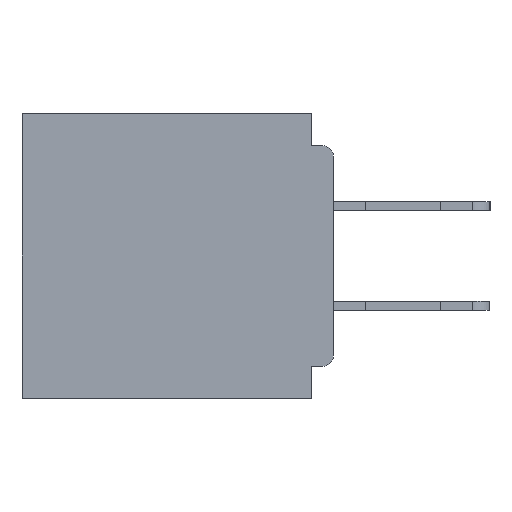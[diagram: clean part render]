
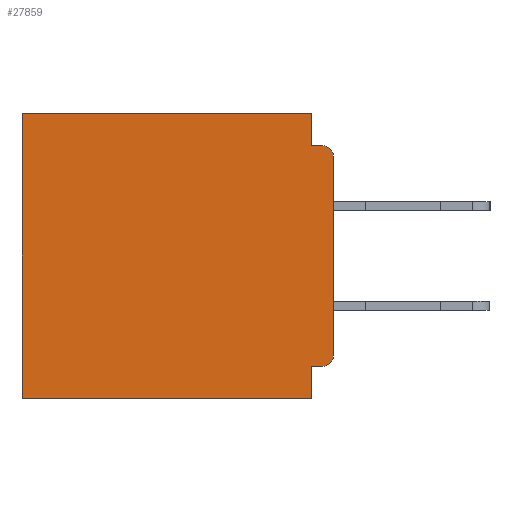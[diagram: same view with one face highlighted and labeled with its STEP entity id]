
A CAD part, left-side view. The second image highlights one B-rep face of the part: STEP entity #27859.
In plain terms, the highlighted planar face has unit normal (-1, 0, 0).
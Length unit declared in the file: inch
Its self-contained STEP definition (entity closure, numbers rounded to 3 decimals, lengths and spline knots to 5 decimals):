
#535 = VECTOR ( 'NONE', #12243, 39.37008 ) ;
#715 = VERTEX_POINT ( 'NONE', #3786 ) ;
#739 = ORIENTED_EDGE ( 'NONE', *, *, #3832, .T. ) ;
#997 = DIRECTION ( 'NONE',  ( 0., 0., -1. ) ) ;
#2430 = ORIENTED_EDGE ( 'NONE', *, *, #18139, .F. ) ;
#3179 = ORIENTED_EDGE ( 'NONE', *, *, #42944, .F. ) ;
#3397 = CARTESIAN_POINT ( 'NONE',  ( 0.3, 0.015, -0.34 ) ) ;
#3786 = CARTESIAN_POINT ( 'NONE',  ( 0.3, 0.031, -0.355 ) ) ;
#3832 = EDGE_CURVE ( 'NONE', #22852, #14120, #15220, .T. ) ;
#4287 = VERTEX_POINT ( 'NONE', #28730 ) ;
#5738 = CARTESIAN_POINT ( 'NONE',  ( 0.3, 0., -0.4 ) ) ;
#5742 = ORIENTED_EDGE ( 'NONE', *, *, #34414, .T. ) ;
#6948 = EDGE_CURVE ( 'NONE', #56632, #6965, #15062, .T. ) ;
#6965 = VERTEX_POINT ( 'NONE', #21066 ) ;
#7620 = LINE ( 'NONE', #5738, #16630 ) ;
#7742 = VECTOR ( 'NONE', #51944, 39.37008 ) ;
#7922 = DIRECTION ( 'NONE',  ( 0., 0., -1. ) ) ;
#9125 = LINE ( 'NONE', #47590, #7742 ) ;
#9281 = FACE_OUTER_BOUND ( 'NONE', #45149, .T. ) ;
#9583 = LINE ( 'NONE', #13804, #41954 ) ;
#9831 = DIRECTION ( 'NONE',  ( 1., 0., 0. ) ) ;
#10188 = DIRECTION ( 'NONE',  ( 0., 0., -1. ) ) ;
#10268 = CARTESIAN_POINT ( 'NONE',  ( 0.3, 0.015, -0.045 ) ) ;
#12243 = DIRECTION ( 'NONE',  ( 0., 0., -1. ) ) ;
#12942 = VERTEX_POINT ( 'NONE', #48364 ) ;
#13123 = AXIS2_PLACEMENT_3D ( 'NONE', #17853, #48549, #22221 ) ;
#13804 = CARTESIAN_POINT ( 'NONE',  ( 0.3, 0., -0.045 ) ) ;
#14120 = VERTEX_POINT ( 'NONE', #25967 ) ;
#15062 = CIRCLE ( 'NONE', #40680, 0.015 ) ;
#15220 = LINE ( 'NONE', #31015, #48896 ) ;
#15748 = ORIENTED_EDGE ( 'NONE', *, *, #42782, .T. ) ;
#16630 = VECTOR ( 'NONE', #10188, 39.37008 ) ;
#17853 = CARTESIAN_POINT ( 'NONE',  ( 0.3, 0.015, -0.06 ) ) ;
#18139 = EDGE_CURVE ( 'NONE', #56632, #715, #43212, .T. ) ;
#18301 = DIRECTION ( 'NONE',  ( 0., -1., 0. ) ) ;
#18500 = CARTESIAN_POINT ( 'NONE',  ( 0.3, 0., -0.355 ) ) ;
#18995 = CARTESIAN_POINT ( 'NONE',  ( 0.3, 0., -0.4 ) ) ;
#20070 = CARTESIAN_POINT ( 'NONE',  ( 0.3, 0.031, 0. ) ) ;
#21066 = CARTESIAN_POINT ( 'NONE',  ( 0.3, 0., -0.34 ) ) ;
#21254 = VERTEX_POINT ( 'NONE', #28806 ) ;
#22221 = DIRECTION ( 'NONE',  ( 0., 0., -1. ) ) ;
#22852 = VERTEX_POINT ( 'NONE', #22892 ) ;
#22892 = CARTESIAN_POINT ( 'NONE',  ( 0.3, 0.437, 0. ) ) ;
#24108 = LINE ( 'NONE', #18995, #44732 ) ;
#25967 = CARTESIAN_POINT ( 'NONE',  ( 0.3, 0.437, -0.4 ) ) ;
#27859 = ADVANCED_FACE ( 'NONE', ( #9281 ), #53790, .F. ) ;
#28730 = CARTESIAN_POINT ( 'NONE',  ( 0.3, 0.031, -0.045 ) ) ;
#28806 = CARTESIAN_POINT ( 'NONE',  ( 0.3, 0.031, -0.4 ) ) ;
#28920 = LINE ( 'NONE', #20070, #39244 ) ;
#31006 = CIRCLE ( 'NONE', #13123, 0.015 ) ;
#31015 = CARTESIAN_POINT ( 'NONE',  ( 0.3, 0.437, -0.4 ) ) ;
#31460 = DIRECTION ( 'NONE',  ( 0., 0., -1. ) ) ;
#31573 = VECTOR ( 'NONE', #40370, 39.37008 ) ;
#33031 = CARTESIAN_POINT ( 'NONE',  ( 0.3, 0.031, 0. ) ) ;
#34342 = DIRECTION ( 'NONE',  ( -1., 0., 0. ) ) ;
#34414 = EDGE_CURVE ( 'NONE', #52807, #22852, #9125, .T. ) ;
#35971 = EDGE_CURVE ( 'NONE', #52807, #4287, #28920, .T. ) ;
#36337 = EDGE_CURVE ( 'NONE', #4287, #50828, #9583, .T. ) ;
#36774 = ORIENTED_EDGE ( 'NONE', *, *, #35971, .F. ) ;
#37721 = DIRECTION ( 'NONE',  ( 0., 0., -1. ) ) ;
#38442 = CARTESIAN_POINT ( 'NONE',  ( 0.3, 0.015, -0.355 ) ) ;
#38523 = ORIENTED_EDGE ( 'NONE', *, *, #36337, .F. ) ;
#39244 = VECTOR ( 'NONE', #37721, 39.37008 ) ;
#40117 = AXIS2_PLACEMENT_3D ( 'NONE', #49453, #9831, #997 ) ;
#40370 = DIRECTION ( 'NONE',  ( 0., 1., 0. ) ) ;
#40680 = AXIS2_PLACEMENT_3D ( 'NONE', #3397, #34342, #7922 ) ;
#41954 = VECTOR ( 'NONE', #18301, 39.37008 ) ;
#42782 = EDGE_CURVE ( 'NONE', #12942, #50828, #31006, .T. ) ;
#42944 = EDGE_CURVE ( 'NONE', #21254, #14120, #24108, .T. ) ;
#43212 = LINE ( 'NONE', #18500, #31573 ) ;
#43599 = EDGE_CURVE ( 'NONE', #12942, #6965, #7620, .T. ) ;
#44732 = VECTOR ( 'NONE', #54015, 39.37008 ) ;
#45149 = EDGE_LOOP ( 'NONE', ( #51095, #15748, #38523, #36774, #5742, #739, #3179, #45948, #2430, #57024 ) ) ;
#45948 = ORIENTED_EDGE ( 'NONE', *, *, #56669, .F. ) ;
#47465 = CARTESIAN_POINT ( 'NONE',  ( 0.3, 0.031, -0.4 ) ) ;
#47527 = LINE ( 'NONE', #47465, #535 ) ;
#47590 = CARTESIAN_POINT ( 'NONE',  ( 0.3, 0., 0. ) ) ;
#48364 = CARTESIAN_POINT ( 'NONE',  ( 0.3, 0., -0.06 ) ) ;
#48549 = DIRECTION ( 'NONE',  ( -1., 0., 0. ) ) ;
#48896 = VECTOR ( 'NONE', #31460, 39.37008 ) ;
#49453 = CARTESIAN_POINT ( 'NONE',  ( 0.3, 0., -0.4 ) ) ;
#50828 = VERTEX_POINT ( 'NONE', #10268 ) ;
#51095 = ORIENTED_EDGE ( 'NONE', *, *, #43599, .F. ) ;
#51944 = DIRECTION ( 'NONE',  ( 0., 1., 0. ) ) ;
#52807 = VERTEX_POINT ( 'NONE', #33031 ) ;
#53790 = PLANE ( 'NONE',  #40117 ) ;
#54015 = DIRECTION ( 'NONE',  ( 0., 1., 0. ) ) ;
#56632 = VERTEX_POINT ( 'NONE', #38442 ) ;
#56669 = EDGE_CURVE ( 'NONE', #715, #21254, #47527, .T. ) ;
#57024 = ORIENTED_EDGE ( 'NONE', *, *, #6948, .T. ) ;
